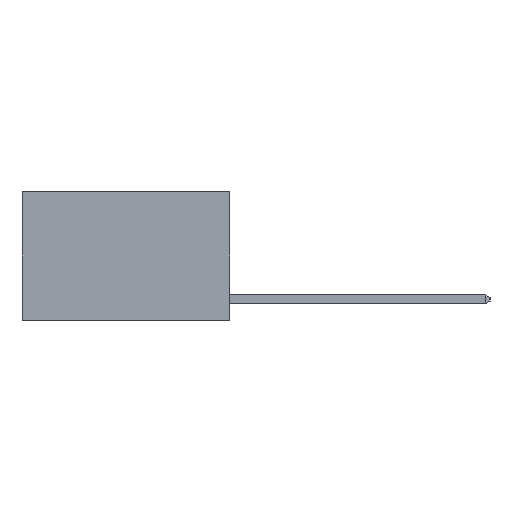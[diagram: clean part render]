
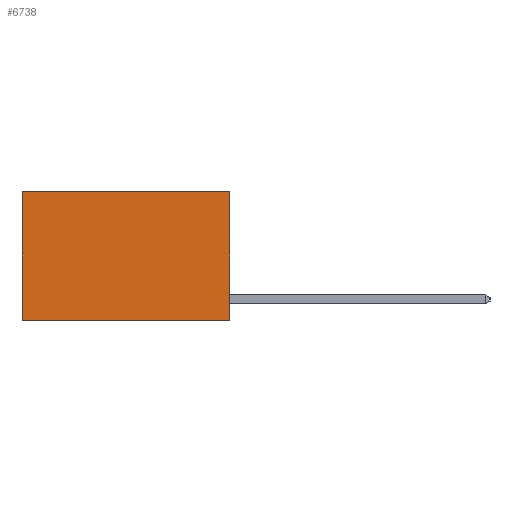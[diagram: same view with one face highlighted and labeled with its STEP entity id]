
A CAD part, left-side view. The second image highlights one B-rep face of the part: STEP entity #6738.
In plain terms, the highlighted planar face has unit normal (-1, 0, 0).
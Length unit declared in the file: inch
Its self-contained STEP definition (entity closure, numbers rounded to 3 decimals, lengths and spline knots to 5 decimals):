
#88 = LINE ( 'NONE', #5133, #11086 ) ;
#180 = CARTESIAN_POINT ( 'NONE',  ( 0.2625, 0., 0. ) ) ;
#322 = LINE ( 'NONE', #7013, #564 ) ;
#346 = VECTOR ( 'NONE', #3627, 39.37008 ) ;
#515 = VERTEX_POINT ( 'NONE', #4868 ) ;
#564 = VECTOR ( 'NONE', #1773, 39.37008 ) ;
#869 = VERTEX_POINT ( 'NONE', #1604 ) ;
#1054 = DIRECTION ( 'NONE',  ( 0., 0., -1. ) ) ;
#1235 = ORIENTED_EDGE ( 'NONE', *, *, #3783, .F. ) ;
#1604 = CARTESIAN_POINT ( 'NONE',  ( 0.2625, 0.6, -0.37 ) ) ;
#1773 = DIRECTION ( 'NONE',  ( 0., 0., -1. ) ) ;
#2684 = CARTESIAN_POINT ( 'NONE',  ( 0.2625, 0.6, 0. ) ) ;
#2763 = ORIENTED_EDGE ( 'NONE', *, *, #9214, .T. ) ;
#2976 = ORIENTED_EDGE ( 'NONE', *, *, #8879, .F. ) ;
#2998 = LINE ( 'NONE', #4532, #346 ) ;
#3530 = VECTOR ( 'NONE', #8419, 39.37008 ) ;
#3627 = DIRECTION ( 'NONE',  ( 0., 0., -1. ) ) ;
#3783 = EDGE_CURVE ( 'NONE', #9226, #869, #88, .T. ) ;
#4307 = DIRECTION ( 'NONE',  ( 0., 1., 0. ) ) ;
#4532 = CARTESIAN_POINT ( 'NONE',  ( 0.2625, 0., 0. ) ) ;
#4615 = PLANE ( 'NONE',  #8810 ) ;
#4868 = CARTESIAN_POINT ( 'NONE',  ( 0.2625, 0., 0. ) ) ;
#5071 = CARTESIAN_POINT ( 'NONE',  ( 0.2625, 0., -0.37 ) ) ;
#5133 = CARTESIAN_POINT ( 'NONE',  ( 0.2625, 0., -0.37 ) ) ;
#5912 = ORIENTED_EDGE ( 'NONE', *, *, #10842, .T. ) ;
#6364 = DIRECTION ( 'NONE',  ( 1., 0., 0. ) ) ;
#6738 = ADVANCED_FACE ( 'NONE', ( #7904 ), #4615, .F. ) ;
#7013 = CARTESIAN_POINT ( 'NONE',  ( 0.2625, 0.6, 0. ) ) ;
#7675 = EDGE_LOOP ( 'NONE', ( #5912, #1235, #2976, #2763 ) ) ;
#7904 = FACE_OUTER_BOUND ( 'NONE', #7675, .T. ) ;
#8419 = DIRECTION ( 'NONE',  ( 0., 1., 0. ) ) ;
#8810 = AXIS2_PLACEMENT_3D ( 'NONE', #180, #6364, #1054 ) ;
#8879 = EDGE_CURVE ( 'NONE', #515, #9226, #2998, .T. ) ;
#9214 = EDGE_CURVE ( 'NONE', #515, #10224, #10083, .T. ) ;
#9226 = VERTEX_POINT ( 'NONE', #5071 ) ;
#10083 = LINE ( 'NONE', #10127, #3530 ) ;
#10127 = CARTESIAN_POINT ( 'NONE',  ( 0.2625, 0., 0. ) ) ;
#10224 = VERTEX_POINT ( 'NONE', #2684 ) ;
#10842 = EDGE_CURVE ( 'NONE', #10224, #869, #322, .T. ) ;
#11086 = VECTOR ( 'NONE', #4307, 39.37008 ) ;
